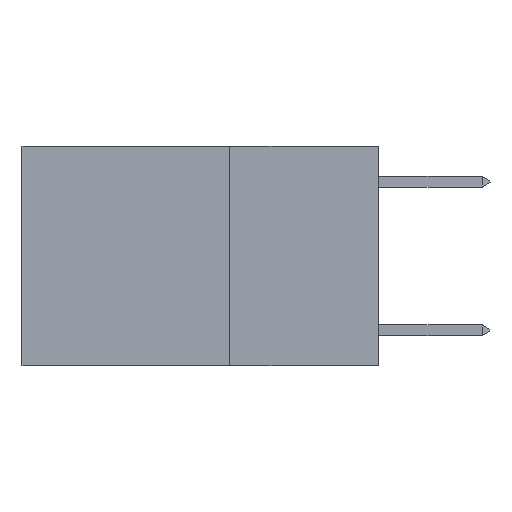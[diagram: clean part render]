
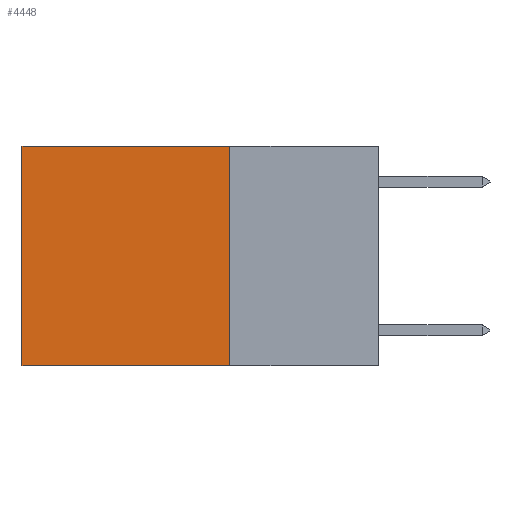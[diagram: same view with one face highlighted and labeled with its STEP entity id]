
A CAD part, left-side view. The second image highlights one B-rep face of the part: STEP entity #4448.
In plain terms, the highlighted planar face has unit normal (-1, 0, 0).
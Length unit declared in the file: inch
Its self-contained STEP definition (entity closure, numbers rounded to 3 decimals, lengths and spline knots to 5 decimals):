
#189 = DIRECTION ( 'NONE',  ( 0., 0., -1. ) ) ;
#657 = ORIENTED_EDGE ( 'NONE', *, *, #12997, .F. ) ;
#816 = FACE_OUTER_BOUND ( 'NONE', #11133, .T. ) ;
#1336 = ORIENTED_EDGE ( 'NONE', *, *, #4153, .T. ) ;
#1952 = EDGE_CURVE ( 'NONE', #6435, #6031, #7341, .T. ) ;
#2237 = CARTESIAN_POINT ( 'NONE',  ( 0.2625, 0.25, -0.37 ) ) ;
#2384 = VECTOR ( 'NONE', #5304, 39.37008 ) ;
#2471 = CARTESIAN_POINT ( 'NONE',  ( 0.2625, 0.6, -0.37 ) ) ;
#3825 = VECTOR ( 'NONE', #7166, 39.37008 ) ;
#3967 = CARTESIAN_POINT ( 'NONE',  ( 0.2625, 0.25, 0. ) ) ;
#4086 = LINE ( 'NONE', #13077, #9406 ) ;
#4153 = EDGE_CURVE ( 'NONE', #6435, #8559, #6638, .T. ) ;
#4400 = PLANE ( 'NONE',  #7872 ) ;
#4448 = ADVANCED_FACE ( 'NONE', ( #816 ), #4400, .F. ) ;
#4580 = CARTESIAN_POINT ( 'NONE',  ( 0.2625, 0.25, 0. ) ) ;
#5304 = DIRECTION ( 'NONE',  ( 0., 0., -1. ) ) ;
#5507 = ORIENTED_EDGE ( 'NONE', *, *, #11992, .T. ) ;
#6031 = VERTEX_POINT ( 'NONE', #6947 ) ;
#6429 = DIRECTION ( 'NONE',  ( 0., 1., 0. ) ) ;
#6435 = VERTEX_POINT ( 'NONE', #4580 ) ;
#6556 = DIRECTION ( 'NONE',  ( 1., 0., 0. ) ) ;
#6638 = LINE ( 'NONE', #3967, #3825 ) ;
#6947 = CARTESIAN_POINT ( 'NONE',  ( 0.2625, 0.25, -0.37 ) ) ;
#7166 = DIRECTION ( 'NONE',  ( 0., 1., 0. ) ) ;
#7341 = LINE ( 'NONE', #11635, #2384 ) ;
#7850 = DIRECTION ( 'NONE',  ( 0., 0., -1. ) ) ;
#7872 = AXIS2_PLACEMENT_3D ( 'NONE', #9723, #6556, #189 ) ;
#8559 = VERTEX_POINT ( 'NONE', #10615 ) ;
#9406 = VECTOR ( 'NONE', #7850, 39.37008 ) ;
#9477 = ORIENTED_EDGE ( 'NONE', *, *, #1952, .F. ) ;
#9723 = CARTESIAN_POINT ( 'NONE',  ( 0.2625, 0.25, 0. ) ) ;
#10615 = CARTESIAN_POINT ( 'NONE',  ( 0.2625, 0.6, 0. ) ) ;
#10621 = VERTEX_POINT ( 'NONE', #2471 ) ;
#11133 = EDGE_LOOP ( 'NONE', ( #5507, #657, #9477, #1336 ) ) ;
#11173 = LINE ( 'NONE', #2237, #13630 ) ;
#11635 = CARTESIAN_POINT ( 'NONE',  ( 0.2625, 0.25, 0. ) ) ;
#11992 = EDGE_CURVE ( 'NONE', #8559, #10621, #4086, .T. ) ;
#12997 = EDGE_CURVE ( 'NONE', #6031, #10621, #11173, .T. ) ;
#13077 = CARTESIAN_POINT ( 'NONE',  ( 0.2625, 0.6, 0. ) ) ;
#13630 = VECTOR ( 'NONE', #6429, 39.37008 ) ;
